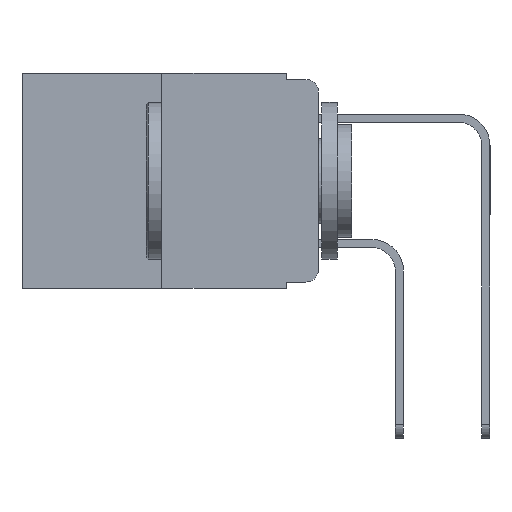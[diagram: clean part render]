
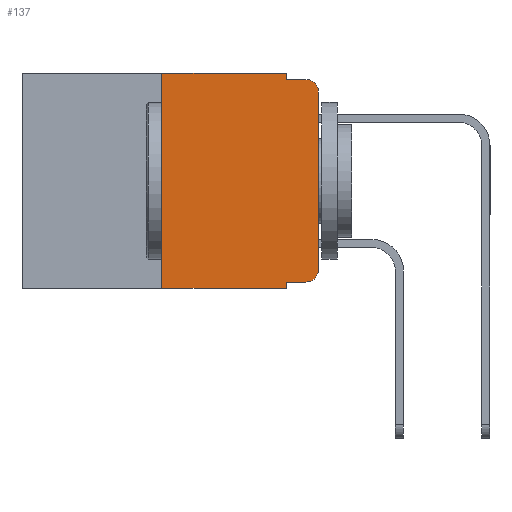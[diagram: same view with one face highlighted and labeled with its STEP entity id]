
A CAD part, left-side view. The second image highlights one B-rep face of the part: STEP entity #137.
In plain terms, the highlighted planar face has unit normal (-1, 0, 0).
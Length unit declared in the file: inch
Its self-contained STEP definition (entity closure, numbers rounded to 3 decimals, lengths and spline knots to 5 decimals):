
#91 = EDGE_CURVE ( 'NONE', #9981, #13420, #17888, .T. ) ;
#137 = ADVANCED_FACE ( 'NONE', ( #9454 ), #17303, .F. ) ;
#975 = CARTESIAN_POINT ( 'NONE',  ( 0., 0.051, 0. ) ) ;
#1079 = ORIENTED_EDGE ( 'NONE', *, *, #10128, .T. ) ;
#1251 = EDGE_CURVE ( 'NONE', #13420, #4469, #10742, .T. ) ;
#1767 = CARTESIAN_POINT ( 'NONE',  ( 0., 0.473, -0.343 ) ) ;
#2134 = ORIENTED_EDGE ( 'NONE', *, *, #8200, .T. ) ;
#2352 = EDGE_CURVE ( 'NONE', #7973, #4469, #14456, .T. ) ;
#2693 = VECTOR ( 'NONE', #15040, 39.37008 ) ;
#2931 = CARTESIAN_POINT ( 'NONE',  ( 0., 0.473, 0. ) ) ;
#2998 = LINE ( 'NONE', #16763, #18150 ) ;
#3036 = CARTESIAN_POINT ( 'NONE',  ( 0., 0., 0. ) ) ;
#3251 = CARTESIAN_POINT ( 'NONE',  ( 0., 0.25, 0. ) ) ;
#3429 = CARTESIAN_POINT ( 'NONE',  ( 0., 0.02, -0.313 ) ) ;
#3431 = EDGE_CURVE ( 'NONE', #15514, #7973, #2998, .T. ) ;
#3478 = VECTOR ( 'NONE', #17482, 39.37008 ) ;
#3551 = VECTOR ( 'NONE', #4419, 39.37008 ) ;
#3828 = CARTESIAN_POINT ( 'NONE',  ( 0., 0.051, -0.333 ) ) ;
#4265 = ORIENTED_EDGE ( 'NONE', *, *, #3431, .F. ) ;
#4381 = EDGE_CURVE ( 'NONE', #10118, #13837, #9994, .T. ) ;
#4419 = DIRECTION ( 'NONE',  ( 0., -1., 0. ) ) ;
#4469 = VERTEX_POINT ( 'NONE', #6343 ) ;
#4701 = DIRECTION ( 'NONE',  ( 0., 0., 1. ) ) ;
#4875 = DIRECTION ( 'NONE',  ( 0., 0., -1. ) ) ;
#5075 = CARTESIAN_POINT ( 'NONE',  ( 0., 0.051, -0.343 ) ) ;
#5236 = VECTOR ( 'NONE', #12284, 39.37008 ) ;
#6287 = DIRECTION ( 'NONE',  ( 0., -1., 0. ) ) ;
#6343 = CARTESIAN_POINT ( 'NONE',  ( 0., 0.02, -0.01 ) ) ;
#6865 = DIRECTION ( 'NONE',  ( 0., 0., -1. ) ) ;
#6950 = VERTEX_POINT ( 'NONE', #16275 ) ;
#6977 = DIRECTION ( 'NONE',  ( 0., 0., -1. ) ) ;
#6987 = DIRECTION ( 'NONE',  ( 0., -1., 0. ) ) ;
#7253 = CARTESIAN_POINT ( 'NONE',  ( 0., 0.051, -0.01 ) ) ;
#7384 = VECTOR ( 'NONE', #6287, 39.37008 ) ;
#7494 = DIRECTION ( 'NONE',  ( 1., 0., 0. ) ) ;
#7574 = CARTESIAN_POINT ( 'NONE',  ( 0., 0.051, -0.333 ) ) ;
#7848 = CARTESIAN_POINT ( 'NONE',  ( 0., 0.02, -0.03 ) ) ;
#7973 = VERTEX_POINT ( 'NONE', #7253 ) ;
#7994 = AXIS2_PLACEMENT_3D ( 'NONE', #7848, #8046, #8004 ) ;
#8004 = DIRECTION ( 'NONE',  ( 0., 0., -1. ) ) ;
#8046 = DIRECTION ( 'NONE',  ( -1., 0., 0. ) ) ;
#8200 = EDGE_CURVE ( 'NONE', #6950, #9981, #13004, .T. ) ;
#8733 = CARTESIAN_POINT ( 'NONE',  ( 0., 0., -0.313 ) ) ;
#9393 = CARTESIAN_POINT ( 'NONE',  ( 0., 0.051, 0. ) ) ;
#9402 = ORIENTED_EDGE ( 'NONE', *, *, #13013, .F. ) ;
#9454 = FACE_OUTER_BOUND ( 'NONE', #11481, .T. ) ;
#9535 = VECTOR ( 'NONE', #4701, 39.37008 ) ;
#9981 = VERTEX_POINT ( 'NONE', #8733 ) ;
#9994 = LINE ( 'NONE', #3251, #9535 ) ;
#10118 = VERTEX_POINT ( 'NONE', #11934 ) ;
#10128 = EDGE_CURVE ( 'NONE', #10118, #12227, #11154, .T. ) ;
#10245 = AXIS2_PLACEMENT_3D ( 'NONE', #3429, #13437, #4875 ) ;
#10651 = EDGE_CURVE ( 'NONE', #13837, #15514, #14939, .T. ) ;
#10675 = VECTOR ( 'NONE', #6987, 39.37008 ) ;
#10742 = CIRCLE ( 'NONE', #7994, 0.02 ) ;
#11063 = LINE ( 'NONE', #7574, #3478 ) ;
#11154 = LINE ( 'NONE', #1767, #7384 ) ;
#11481 = EDGE_LOOP ( 'NONE', ( #14763, #18465, #15206, #4265, #11876, #16080, #1079, #9402, #16938, #2134 ) ) ;
#11876 = ORIENTED_EDGE ( 'NONE', *, *, #10651, .F. ) ;
#11934 = CARTESIAN_POINT ( 'NONE',  ( 0., 0.25, -0.343 ) ) ;
#12040 = EDGE_CURVE ( 'NONE', #18352, #6950, #11063, .T. ) ;
#12227 = VERTEX_POINT ( 'NONE', #5075 ) ;
#12284 = DIRECTION ( 'NONE',  ( 0., 0., -1. ) ) ;
#12589 = CARTESIAN_POINT ( 'NONE',  ( 0., 0., -0.03 ) ) ;
#12837 = LINE ( 'NONE', #9393, #5236 ) ;
#13004 = CIRCLE ( 'NONE', #10245, 0.02 ) ;
#13013 = EDGE_CURVE ( 'NONE', #18352, #12227, #12837, .T. ) ;
#13271 = CARTESIAN_POINT ( 'NONE',  ( 0., 0.473, 0. ) ) ;
#13406 = CARTESIAN_POINT ( 'NONE',  ( 0., 0.051, -0.01 ) ) ;
#13420 = VERTEX_POINT ( 'NONE', #12589 ) ;
#13437 = DIRECTION ( 'NONE',  ( -1., 0., 0. ) ) ;
#13837 = VERTEX_POINT ( 'NONE', #16269 ) ;
#14456 = LINE ( 'NONE', #13406, #10675 ) ;
#14763 = ORIENTED_EDGE ( 'NONE', *, *, #91, .T. ) ;
#14939 = LINE ( 'NONE', #2931, #3551 ) ;
#15040 = DIRECTION ( 'NONE',  ( 0., 0., 1. ) ) ;
#15206 = ORIENTED_EDGE ( 'NONE', *, *, #2352, .F. ) ;
#15514 = VERTEX_POINT ( 'NONE', #975 ) ;
#16080 = ORIENTED_EDGE ( 'NONE', *, *, #4381, .F. ) ;
#16269 = CARTESIAN_POINT ( 'NONE',  ( 0., 0.25, 0. ) ) ;
#16275 = CARTESIAN_POINT ( 'NONE',  ( 0., 0.02, -0.333 ) ) ;
#16763 = CARTESIAN_POINT ( 'NONE',  ( 0., 0.051, 0. ) ) ;
#16938 = ORIENTED_EDGE ( 'NONE', *, *, #12040, .T. ) ;
#17303 = PLANE ( 'NONE',  #17358 ) ;
#17358 = AXIS2_PLACEMENT_3D ( 'NONE', #13271, #7494, #6977 ) ;
#17482 = DIRECTION ( 'NONE',  ( 0., -1., 0. ) ) ;
#17888 = LINE ( 'NONE', #3036, #2693 ) ;
#18150 = VECTOR ( 'NONE', #6865, 39.37008 ) ;
#18352 = VERTEX_POINT ( 'NONE', #3828 ) ;
#18465 = ORIENTED_EDGE ( 'NONE', *, *, #1251, .T. ) ;
